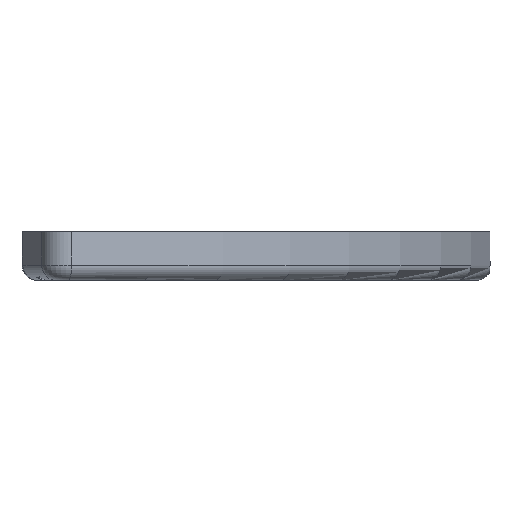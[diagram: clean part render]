
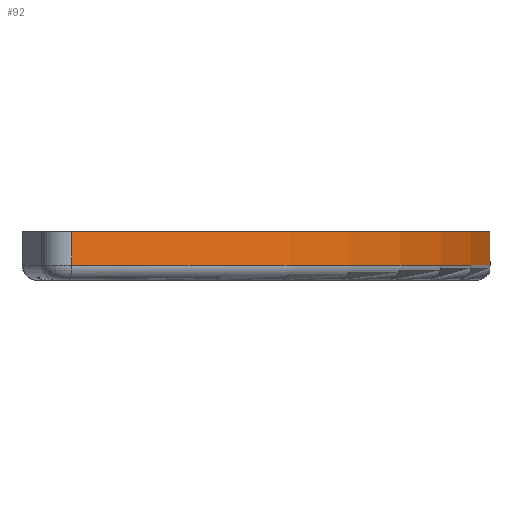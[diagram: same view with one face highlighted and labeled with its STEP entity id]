
A CAD part, front view. The second image highlights one B-rep face of the part: STEP entity #92.
In plain terms, the highlighted cylindrical face has radius 195 mm (diameter 390 mm), a partial arc.
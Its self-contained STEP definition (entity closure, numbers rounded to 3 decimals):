
#86 = DIRECTION ( 'NONE',  ( 0., 0., 1. ) ) ;
#92 = ADVANCED_FACE ( 'NONE', ( #2156 ), #2818, .T. ) ;
#176 = ORIENTED_EDGE ( 'NONE', *, *, #2720, .F. ) ;
#318 = CARTESIAN_POINT ( 'NONE',  ( 17.505, -31.094, -17.6 ) ) ;
#386 = EDGE_LOOP ( 'NONE', ( #880, #2065, #176, #1376 ) ) ;
#387 = VECTOR ( 'NONE', #1991, 1000. ) ;
#456 = AXIS2_PLACEMENT_3D ( 'NONE', #1597, #2527, #2547 ) ;
#566 = DIRECTION ( 'NONE',  ( 0., 0., 1. ) ) ;
#615 = VERTEX_POINT ( 'NONE', #1739 ) ;
#672 = EDGE_CURVE ( 'NONE', #615, #1427, #1009, .T. ) ;
#781 = VERTEX_POINT ( 'NONE', #955 ) ;
#797 = DIRECTION ( 'NONE',  ( 0., 0., 1. ) ) ;
#815 = EDGE_CURVE ( 'NONE', #781, #1593, #1987, .T. ) ;
#880 = ORIENTED_EDGE ( 'NONE', *, *, #1478, .T. ) ;
#955 = CARTESIAN_POINT ( 'NONE',  ( 17.505, -31.094, -11. ) ) ;
#989 = CARTESIAN_POINT ( 'NONE',  ( 17.505, -31.094, 0. ) ) ;
#1009 = LINE ( 'NONE', #2194, #387 ) ;
#1224 = CARTESIAN_POINT ( 'NONE',  ( -120.513, -187.233, -11. ) ) ;
#1376 = ORIENTED_EDGE ( 'NONE', *, *, #672, .T. ) ;
#1427 = VERTEX_POINT ( 'NONE', #1224 ) ;
#1478 = EDGE_CURVE ( 'NONE', #1427, #781, #1621, .T. ) ;
#1479 = CARTESIAN_POINT ( 'NONE',  ( -175., 0., -11. ) ) ;
#1593 = VERTEX_POINT ( 'NONE', #989 ) ;
#1597 = CARTESIAN_POINT ( 'NONE',  ( -175., 0., -17.6 ) ) ;
#1621 = CIRCLE ( 'NONE', #2624, 195. ) ;
#1707 = DIRECTION ( 'NONE',  ( 1., 0., 0. ) ) ;
#1739 = CARTESIAN_POINT ( 'NONE',  ( -120.513, -187.233, 0. ) ) ;
#1828 = VECTOR ( 'NONE', #797, 1000. ) ;
#1955 = CARTESIAN_POINT ( 'NONE',  ( -175., 0., 0. ) ) ;
#1987 = LINE ( 'NONE', #318, #1828 ) ;
#1991 = DIRECTION ( 'NONE',  ( 0., 0., -1. ) ) ;
#2065 = ORIENTED_EDGE ( 'NONE', *, *, #815, .T. ) ;
#2156 = FACE_OUTER_BOUND ( 'NONE', #386, .T. ) ;
#2183 = DIRECTION ( 'NONE',  ( 1., 0., 0. ) ) ;
#2194 = CARTESIAN_POINT ( 'NONE',  ( -120.513, -187.233, -17.6 ) ) ;
#2202 = CIRCLE ( 'NONE', #2278, 195. ) ;
#2278 = AXIS2_PLACEMENT_3D ( 'NONE', #1955, #566, #2183 ) ;
#2527 = DIRECTION ( 'NONE',  ( 0., 0., 1. ) ) ;
#2547 = DIRECTION ( 'NONE',  ( 1., 0., 0. ) ) ;
#2624 = AXIS2_PLACEMENT_3D ( 'NONE', #1479, #86, #1707 ) ;
#2720 = EDGE_CURVE ( 'NONE', #615, #1593, #2202, .T. ) ;
#2818 = CYLINDRICAL_SURFACE ( 'NONE', #456, 195. ) ;
